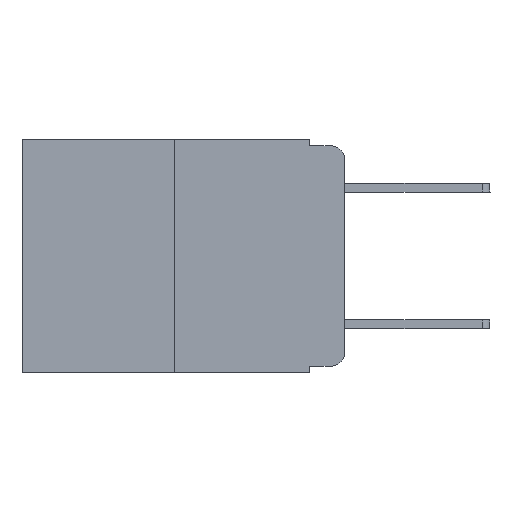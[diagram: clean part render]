
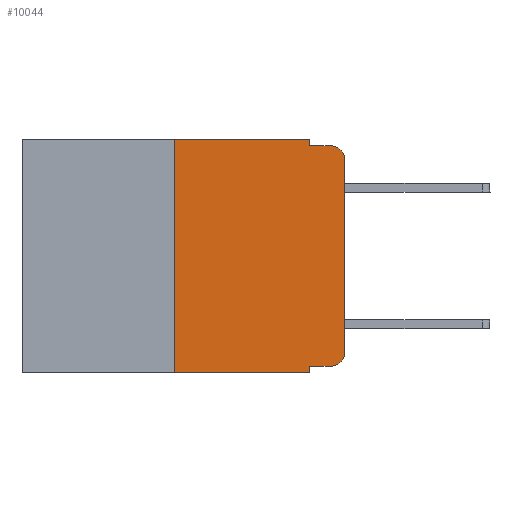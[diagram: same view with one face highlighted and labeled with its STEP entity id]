
A CAD part, left-side view. The second image highlights one B-rep face of the part: STEP entity #10044.
In plain terms, the highlighted planar face has unit normal (-1, 0, 0).
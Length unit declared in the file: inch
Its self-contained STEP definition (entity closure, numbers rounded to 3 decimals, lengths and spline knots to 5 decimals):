
#355 = FACE_OUTER_BOUND ( 'NONE', #5648, .T. ) ;
#472 = VECTOR ( 'NONE', #3567, 39.37008 ) ;
#1080 = ORIENTED_EDGE ( 'NONE', *, *, #9924, .F. ) ;
#1502 = DIRECTION ( 'NONE',  ( 0., 0., -1. ) ) ;
#1698 = LINE ( 'NONE', #22026, #12859 ) ;
#1708 = VERTEX_POINT ( 'NONE', #17369 ) ;
#1978 = AXIS2_PLACEMENT_3D ( 'NONE', #18133, #23925, #1502 ) ;
#2132 = VERTEX_POINT ( 'NONE', #5981 ) ;
#2994 = EDGE_CURVE ( 'NONE', #2132, #3868, #11724, .T. ) ;
#3567 = DIRECTION ( 'NONE',  ( 0., -1., 0. ) ) ;
#3868 = VERTEX_POINT ( 'NONE', #3893 ) ;
#3886 = AXIS2_PLACEMENT_3D ( 'NONE', #7852, #22271, #16966 ) ;
#3893 = CARTESIAN_POINT ( 'NONE',  ( 0., 0., -0.03 ) ) ;
#4177 = ORIENTED_EDGE ( 'NONE', *, *, #14609, .T. ) ;
#4580 = CARTESIAN_POINT ( 'NONE',  ( 0., 0.25, 0. ) ) ;
#4595 = DIRECTION ( 'NONE',  ( 0., 0., -1. ) ) ;
#4675 = ORIENTED_EDGE ( 'NONE', *, *, #2994, .T. ) ;
#5648 = EDGE_LOOP ( 'NONE', ( #4675, #21193, #7157, #14273, #24040, #17199, #8668, #1080, #4177, #14611 ) ) ;
#5865 = EDGE_CURVE ( 'NONE', #7516, #15173, #1698, .T. ) ;
#5981 = CARTESIAN_POINT ( 'NONE',  ( 0., 0., -0.313 ) ) ;
#6260 = CARTESIAN_POINT ( 'NONE',  ( 0., 0.473, 0. ) ) ;
#6389 = LINE ( 'NONE', #6260, #19739 ) ;
#6664 = CARTESIAN_POINT ( 'NONE',  ( 0., 0.051, 0. ) ) ;
#6988 = CARTESIAN_POINT ( 'NONE',  ( 0., 0.02, -0.313 ) ) ;
#7157 = ORIENTED_EDGE ( 'NONE', *, *, #5865, .F. ) ;
#7203 = CARTESIAN_POINT ( 'NONE',  ( 0., 0.051, 0. ) ) ;
#7516 = VERTEX_POINT ( 'NONE', #8957 ) ;
#7852 = CARTESIAN_POINT ( 'NONE',  ( 0., 0.473, 0. ) ) ;
#8053 = EDGE_CURVE ( 'NONE', #1708, #23667, #15548, .T. ) ;
#8136 = DIRECTION ( 'NONE',  ( 0., 0., 1. ) ) ;
#8564 = VERTEX_POINT ( 'NONE', #10103 ) ;
#8668 = ORIENTED_EDGE ( 'NONE', *, *, #23590, .T. ) ;
#8759 = LINE ( 'NONE', #16630, #472 ) ;
#8957 = CARTESIAN_POINT ( 'NONE',  ( 0., 0.051, -0.01 ) ) ;
#9924 = EDGE_CURVE ( 'NONE', #8564, #14088, #10379, .T. ) ;
#9988 = LINE ( 'NONE', #12078, #23713 ) ;
#10044 = ADVANCED_FACE ( 'NONE', ( #355 ), #11208, .F. ) ;
#10103 = CARTESIAN_POINT ( 'NONE',  ( 0., 0.051, -0.333 ) ) ;
#10379 = LINE ( 'NONE', #15918, #18819 ) ;
#10500 = DIRECTION ( 'NONE',  ( 0., 0., -1. ) ) ;
#10886 = VECTOR ( 'NONE', #8136, 39.37008 ) ;
#10920 = VERTEX_POINT ( 'NONE', #15072 ) ;
#11208 = PLANE ( 'NONE',  #3886 ) ;
#11724 = LINE ( 'NONE', #19086, #10886 ) ;
#12078 = CARTESIAN_POINT ( 'NONE',  ( 0., 0.473, -0.343 ) ) ;
#12102 = DIRECTION ( 'NONE',  ( 0., 0., 1. ) ) ;
#12436 = DIRECTION ( 'NONE',  ( -1., 0., 0. ) ) ;
#12859 = VECTOR ( 'NONE', #20188, 39.37008 ) ;
#14088 = VERTEX_POINT ( 'NONE', #24036 ) ;
#14273 = ORIENTED_EDGE ( 'NONE', *, *, #19840, .F. ) ;
#14512 = DIRECTION ( 'NONE',  ( 0., 0., -1. ) ) ;
#14609 = EDGE_CURVE ( 'NONE', #8564, #10920, #8759, .T. ) ;
#14611 = ORIENTED_EDGE ( 'NONE', *, *, #17298, .T. ) ;
#15072 = CARTESIAN_POINT ( 'NONE',  ( 0., 0.02, -0.333 ) ) ;
#15173 = VERTEX_POINT ( 'NONE', #17416 ) ;
#15548 = LINE ( 'NONE', #4580, #17635 ) ;
#15918 = CARTESIAN_POINT ( 'NONE',  ( 0., 0.051, 0. ) ) ;
#16290 = LINE ( 'NONE', #6664, #18990 ) ;
#16429 = VERTEX_POINT ( 'NONE', #7203 ) ;
#16630 = CARTESIAN_POINT ( 'NONE',  ( 0., 0.051, -0.333 ) ) ;
#16966 = DIRECTION ( 'NONE',  ( 0., 0., -1. ) ) ;
#17033 = EDGE_CURVE ( 'NONE', #23667, #16429, #6389, .T. ) ;
#17199 = ORIENTED_EDGE ( 'NONE', *, *, #8053, .F. ) ;
#17298 = EDGE_CURVE ( 'NONE', #10920, #2132, #17383, .T. ) ;
#17369 = CARTESIAN_POINT ( 'NONE',  ( 0., 0.25, -0.343 ) ) ;
#17383 = CIRCLE ( 'NONE', #23674, 0.02 ) ;
#17416 = CARTESIAN_POINT ( 'NONE',  ( 0., 0.02, -0.01 ) ) ;
#17635 = VECTOR ( 'NONE', #12102, 39.37008 ) ;
#17720 = DIRECTION ( 'NONE',  ( 0., -1., 0. ) ) ;
#18133 = CARTESIAN_POINT ( 'NONE',  ( 0., 0.02, -0.03 ) ) ;
#18819 = VECTOR ( 'NONE', #10500, 39.37008 ) ;
#18990 = VECTOR ( 'NONE', #4595, 39.37008 ) ;
#19086 = CARTESIAN_POINT ( 'NONE',  ( 0., 0., 0. ) ) ;
#19739 = VECTOR ( 'NONE', #23395, 39.37008 ) ;
#19840 = EDGE_CURVE ( 'NONE', #16429, #7516, #16290, .T. ) ;
#20188 = DIRECTION ( 'NONE',  ( 0., -1., 0. ) ) ;
#20479 = CIRCLE ( 'NONE', #1978, 0.02 ) ;
#20953 = CARTESIAN_POINT ( 'NONE',  ( 0., 0.25, 0. ) ) ;
#21193 = ORIENTED_EDGE ( 'NONE', *, *, #21603, .T. ) ;
#21603 = EDGE_CURVE ( 'NONE', #3868, #15173, #20479, .T. ) ;
#22026 = CARTESIAN_POINT ( 'NONE',  ( 0., 0.051, -0.01 ) ) ;
#22271 = DIRECTION ( 'NONE',  ( 1., 0., 0. ) ) ;
#23395 = DIRECTION ( 'NONE',  ( 0., -1., 0. ) ) ;
#23590 = EDGE_CURVE ( 'NONE', #1708, #14088, #9988, .T. ) ;
#23667 = VERTEX_POINT ( 'NONE', #20953 ) ;
#23674 = AXIS2_PLACEMENT_3D ( 'NONE', #6988, #12436, #14512 ) ;
#23713 = VECTOR ( 'NONE', #17720, 39.37008 ) ;
#23925 = DIRECTION ( 'NONE',  ( -1., 0., 0. ) ) ;
#24036 = CARTESIAN_POINT ( 'NONE',  ( 0., 0.051, -0.343 ) ) ;
#24040 = ORIENTED_EDGE ( 'NONE', *, *, #17033, .F. ) ;
